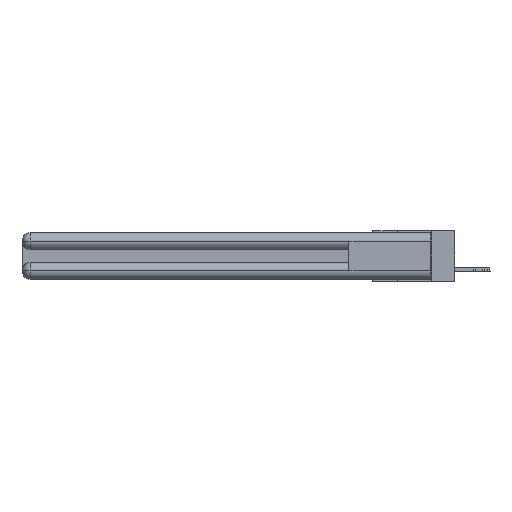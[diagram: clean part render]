
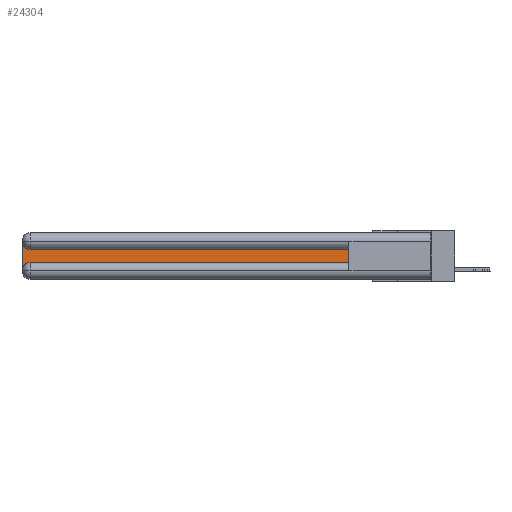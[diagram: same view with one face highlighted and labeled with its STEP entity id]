
A CAD part, left-side view. The second image highlights one B-rep face of the part: STEP entity #24304.
In plain terms, the highlighted planar face has unit normal (-1, 0, 0).
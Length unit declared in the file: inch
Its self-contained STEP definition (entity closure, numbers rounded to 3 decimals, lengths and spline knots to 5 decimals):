
#1030 = CARTESIAN_POINT ( 'NONE',  ( 0.075, 2.94, -0.2175 ) ) ;
#2510 = PLANE ( 'NONE',  #7704 ) ;
#2555 = DIRECTION ( 'NONE',  ( 1., 0., 0. ) ) ;
#2820 = ORIENTED_EDGE ( 'NONE', *, *, #24987, .T. ) ;
#3325 = EDGE_LOOP ( 'NONE', ( #5721, #6716, #13453, #22089, #2820, #14563 ) ) ;
#4471 = CARTESIAN_POINT ( 'NONE',  ( 0.075, 0.6, -0.2175 ) ) ;
#5108 = VERTEX_POINT ( 'NONE', #12937 ) ;
#5286 = FACE_OUTER_BOUND ( 'NONE', #3325, .T. ) ;
#5721 = ORIENTED_EDGE ( 'NONE', *, *, #5849, .T. ) ;
#5849 = EDGE_CURVE ( 'NONE', #17885, #5108, #19902, .T. ) ;
#5868 = DIRECTION ( 'NONE',  ( 0., 0., -1. ) ) ;
#6312 = CIRCLE ( 'NONE', #29058, 0.06 ) ;
#6716 = ORIENTED_EDGE ( 'NONE', *, *, #18426, .T. ) ;
#7704 = AXIS2_PLACEMENT_3D ( 'NONE', #29693, #9840, #12003 ) ;
#8530 = CARTESIAN_POINT ( 'NONE',  ( 0.075, 3., -0.2775 ) ) ;
#9840 = DIRECTION ( 'NONE',  ( 1., 0., 0. ) ) ;
#10374 = DIRECTION ( 'NONE',  ( 0., 0., 1. ) ) ;
#11234 = LINE ( 'NONE', #25114, #29465 ) ;
#11894 = AXIS2_PLACEMENT_3D ( 'NONE', #24836, #2555, #25157 ) ;
#12003 = DIRECTION ( 'NONE',  ( 0., 0., -1. ) ) ;
#12375 = DIRECTION ( 'NONE',  ( 0., 0., -1. ) ) ;
#12867 = EDGE_CURVE ( 'NONE', #31415, #30725, #6312, .T. ) ;
#12937 = CARTESIAN_POINT ( 'NONE',  ( 0.075, 2.94, -0.1225 ) ) ;
#13318 = CARTESIAN_POINT ( 'NONE',  ( 0.075, 0.6, -0.1225 ) ) ;
#13453 = ORIENTED_EDGE ( 'NONE', *, *, #25464, .T. ) ;
#14563 = ORIENTED_EDGE ( 'NONE', *, *, #22440, .T. ) ;
#17060 = CARTESIAN_POINT ( 'NONE',  ( 0.075, 2.94, -0.2775 ) ) ;
#17219 = VECTOR ( 'NONE', #5868, 39.37008 ) ;
#17885 = VERTEX_POINT ( 'NONE', #31041 ) ;
#18199 = CARTESIAN_POINT ( 'NONE',  ( 0.075, 3., -0.2175 ) ) ;
#18426 = EDGE_CURVE ( 'NONE', #5108, #28916, #28794, .T. ) ;
#19176 = LINE ( 'NONE', #24192, #24975 ) ;
#19883 = DIRECTION ( 'NONE',  ( 1., 0., 0. ) ) ;
#19902 = LINE ( 'NONE', #13318, #30747 ) ;
#22089 = ORIENTED_EDGE ( 'NONE', *, *, #12867, .T. ) ;
#22440 = EDGE_CURVE ( 'NONE', #24185, #17885, #11234, .T. ) ;
#24085 = DIRECTION ( 'NONE',  ( 0., -1., 0. ) ) ;
#24185 = VERTEX_POINT ( 'NONE', #4471 ) ;
#24192 = CARTESIAN_POINT ( 'NONE',  ( 0.075, 0.6, -0.2175 ) ) ;
#24304 = ADVANCED_FACE ( 'NONE', ( #5286 ), #2510, .F. ) ;
#24836 = CARTESIAN_POINT ( 'NONE',  ( 0.075, 2.94, -0.0625 ) ) ;
#24975 = VECTOR ( 'NONE', #24085, 39.37008 ) ;
#24987 = EDGE_CURVE ( 'NONE', #30725, #24185, #19176, .T. ) ;
#25114 = CARTESIAN_POINT ( 'NONE',  ( 0.075, 0.6, -0.2175 ) ) ;
#25157 = DIRECTION ( 'NONE',  ( 0., 0., -1. ) ) ;
#25464 = EDGE_CURVE ( 'NONE', #28916, #31415, #30780, .T. ) ;
#28794 = CIRCLE ( 'NONE', #11894, 0.06 ) ;
#28916 = VERTEX_POINT ( 'NONE', #29845 ) ;
#29058 = AXIS2_PLACEMENT_3D ( 'NONE', #17060, #19883, #12375 ) ;
#29465 = VECTOR ( 'NONE', #10374, 39.37008 ) ;
#29693 = CARTESIAN_POINT ( 'NONE',  ( 0.075, 3., -0.1225 ) ) ;
#29845 = CARTESIAN_POINT ( 'NONE',  ( 0.075, 3., -0.0625 ) ) ;
#30725 = VERTEX_POINT ( 'NONE', #1030 ) ;
#30747 = VECTOR ( 'NONE', #30776, 39.37008 ) ;
#30776 = DIRECTION ( 'NONE',  ( 0., 1., 0. ) ) ;
#30780 = LINE ( 'NONE', #18199, #17219 ) ;
#31041 = CARTESIAN_POINT ( 'NONE',  ( 0.075, 0.6, -0.1225 ) ) ;
#31415 = VERTEX_POINT ( 'NONE', #8530 ) ;
